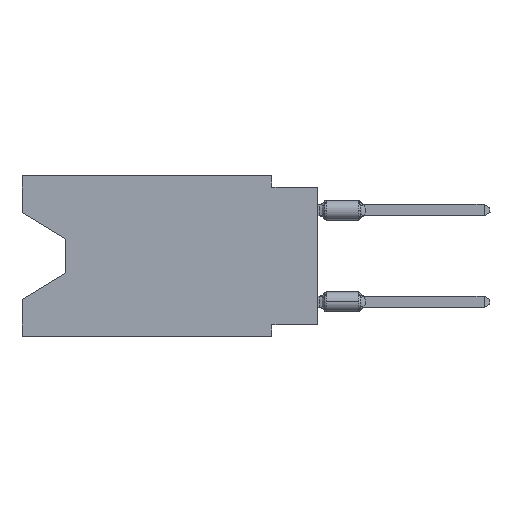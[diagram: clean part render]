
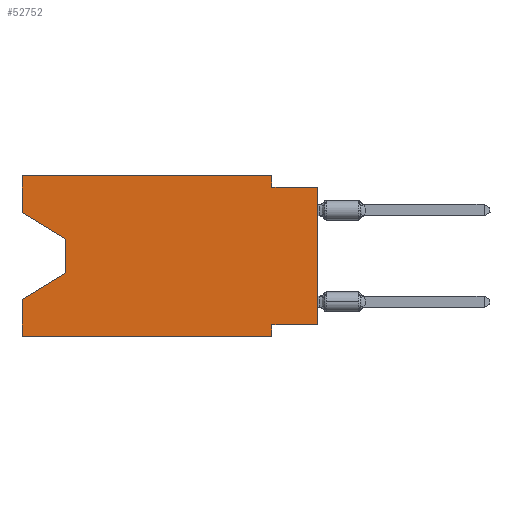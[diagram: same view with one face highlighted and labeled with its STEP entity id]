
A CAD part, left-side view. The second image highlights one B-rep face of the part: STEP entity #52752.
In plain terms, the highlighted planar face has unit normal (-1, 0, 0).
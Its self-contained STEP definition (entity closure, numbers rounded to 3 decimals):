
#1419 = VERTEX_POINT ( 'NONE', #22044 ) ;
#2936 = EDGE_CURVE ( 'NONE', #29716, #54374, #55581, .T. ) ;
#2951 = CARTESIAN_POINT ( 'NONE',  ( 0., 16.383, 0. ) ) ;
#3205 = VECTOR ( 'NONE', #17647, 1000. ) ;
#3366 = CARTESIAN_POINT ( 'NONE',  ( 0., 16.383, -8.89 ) ) ;
#3474 = LINE ( 'NONE', #35937, #59572 ) ;
#4101 = EDGE_CURVE ( 'NONE', #14996, #55507, #55052, .T. ) ;
#4157 = CARTESIAN_POINT ( 'NONE',  ( 0., 2.54, -8.89 ) ) ;
#6747 = ORIENTED_EDGE ( 'NONE', *, *, #42123, .F. ) ;
#6949 = ORIENTED_EDGE ( 'NONE', *, *, #49594, .F. ) ;
#8216 = EDGE_LOOP ( 'NONE', ( #9287, #29771, #29939, #52723, #46484, #22225, #6949, #10009, #47069, #6747, #33922, #58897 ) ) ;
#8384 = FACE_OUTER_BOUND ( 'NONE', #8216, .T. ) ;
#9071 = VECTOR ( 'NONE', #35763, 1000. ) ;
#9287 = ORIENTED_EDGE ( 'NONE', *, *, #38627, .T. ) ;
#10009 = ORIENTED_EDGE ( 'NONE', *, *, #59670, .T. ) ;
#11214 = EDGE_CURVE ( 'NONE', #1419, #29716, #36319, .T. ) ;
#11278 = CARTESIAN_POINT ( 'NONE',  ( 0., 16.383, -8.89 ) ) ;
#12383 = CARTESIAN_POINT ( 'NONE',  ( 0., 2.54, -8.255 ) ) ;
#12990 = LINE ( 'NONE', #50247, #9071 ) ;
#13232 = DIRECTION ( 'NONE',  ( 0., 0., -1. ) ) ;
#13260 = DIRECTION ( 'NONE',  ( 0., 0., 1. ) ) ;
#13549 = CARTESIAN_POINT ( 'NONE',  ( 0., 0., -0.635 ) ) ;
#14455 = EDGE_CURVE ( 'NONE', #52986, #44238, #45211, .T. ) ;
#14996 = VERTEX_POINT ( 'NONE', #30205 ) ;
#15705 = DIRECTION ( 'NONE',  ( 0., 0., -1. ) ) ;
#15811 = VERTEX_POINT ( 'NONE', #12383 ) ;
#16048 = VECTOR ( 'NONE', #13260, 1000. ) ;
#17647 = DIRECTION ( 'NONE',  ( 0., 0.855, -0.519 ) ) ;
#17855 = AXIS2_PLACEMENT_3D ( 'NONE', #44449, #21429, #13232 ) ;
#18126 = VERTEX_POINT ( 'NONE', #3366 ) ;
#18616 = VERTEX_POINT ( 'NONE', #4157 ) ;
#19093 = VECTOR ( 'NONE', #15705, 1000. ) ;
#19502 = CARTESIAN_POINT ( 'NONE',  ( 0., 16.383, -2.038 ) ) ;
#19797 = DIRECTION ( 'NONE',  ( 0., -0.855, -0.519 ) ) ;
#19832 = EDGE_CURVE ( 'NONE', #38888, #52986, #32906, .T. ) ;
#21429 = DIRECTION ( 'NONE',  ( 1., 0., 0. ) ) ;
#22044 = CARTESIAN_POINT ( 'NONE',  ( 0., 16.383, -2.038 ) ) ;
#22225 = ORIENTED_EDGE ( 'NONE', *, *, #54129, .F. ) ;
#22318 = PLANE ( 'NONE',  #17855 ) ;
#24357 = VECTOR ( 'NONE', #51919, 1000. ) ;
#25204 = DIRECTION ( 'NONE',  ( 0., -1., 0. ) ) ;
#26880 = VECTOR ( 'NONE', #25204, 1000. ) ;
#28217 = EDGE_CURVE ( 'NONE', #18126, #18616, #33749, .T. ) ;
#28597 = LINE ( 'NONE', #19502, #48849 ) ;
#28712 = VECTOR ( 'NONE', #47678, 1000. ) ;
#29716 = VERTEX_POINT ( 'NONE', #40355 ) ;
#29771 = ORIENTED_EDGE ( 'NONE', *, *, #19832, .T. ) ;
#29939 = ORIENTED_EDGE ( 'NONE', *, *, #14455, .T. ) ;
#30187 = CARTESIAN_POINT ( 'NONE',  ( 0., 13.97, -5.385 ) ) ;
#30205 = CARTESIAN_POINT ( 'NONE',  ( 0., 2.54, -0.635 ) ) ;
#32906 = LINE ( 'NONE', #33200, #28712 ) ;
#33200 = CARTESIAN_POINT ( 'NONE',  ( 0., 13.97, -3.505 ) ) ;
#33749 = LINE ( 'NONE', #11278, #26880 ) ;
#33922 = ORIENTED_EDGE ( 'NONE', *, *, #2936, .F. ) ;
#34188 = VECTOR ( 'NONE', #35529, 1000. ) ;
#35529 = DIRECTION ( 'NONE',  ( 0., 0., 1. ) ) ;
#35763 = DIRECTION ( 'NONE',  ( 0., 0., 1. ) ) ;
#35937 = CARTESIAN_POINT ( 'NONE',  ( 0., 2.54, -8.89 ) ) ;
#36319 = LINE ( 'NONE', #2951, #16048 ) ;
#37461 = CARTESIAN_POINT ( 'NONE',  ( 0., 0., -0.635 ) ) ;
#38627 = EDGE_CURVE ( 'NONE', #1419, #38888, #28597, .T. ) ;
#38888 = VERTEX_POINT ( 'NONE', #46308 ) ;
#39053 = LINE ( 'NONE', #39938, #53126 ) ;
#39938 = CARTESIAN_POINT ( 'NONE',  ( 0., 0., -8.255 ) ) ;
#40355 = CARTESIAN_POINT ( 'NONE',  ( 0., 16.383, 0. ) ) ;
#42039 = DIRECTION ( 'NONE',  ( 0., -1., 0. ) ) ;
#42123 = EDGE_CURVE ( 'NONE', #54374, #14996, #43880, .T. ) ;
#42581 = CARTESIAN_POINT ( 'NONE',  ( 0., 0., -8.255 ) ) ;
#43661 = EDGE_CURVE ( 'NONE', #18126, #44238, #12990, .T. ) ;
#43692 = CARTESIAN_POINT ( 'NONE',  ( 0., 0., 0. ) ) ;
#43880 = LINE ( 'NONE', #57215, #19093 ) ;
#44238 = VERTEX_POINT ( 'NONE', #51381 ) ;
#44449 = CARTESIAN_POINT ( 'NONE',  ( 0., 16.383, 0. ) ) ;
#45211 = LINE ( 'NONE', #30187, #3205 ) ;
#46308 = CARTESIAN_POINT ( 'NONE',  ( 0., 13.97, -3.505 ) ) ;
#46477 = CARTESIAN_POINT ( 'NONE',  ( 0., 16.383, 0. ) ) ;
#46484 = ORIENTED_EDGE ( 'NONE', *, *, #28217, .T. ) ;
#47069 = ORIENTED_EDGE ( 'NONE', *, *, #4101, .F. ) ;
#47678 = DIRECTION ( 'NONE',  ( 0., 0., -1. ) ) ;
#48849 = VECTOR ( 'NONE', #19797, 1000. ) ;
#49594 = EDGE_CURVE ( 'NONE', #56986, #15811, #39053, .T. ) ;
#50247 = CARTESIAN_POINT ( 'NONE',  ( 0., 16.383, 0. ) ) ;
#51381 = CARTESIAN_POINT ( 'NONE',  ( 0., 16.383, -6.852 ) ) ;
#51919 = DIRECTION ( 'NONE',  ( 0., -1., 0. ) ) ;
#52723 = ORIENTED_EDGE ( 'NONE', *, *, #43661, .F. ) ;
#52752 = ADVANCED_FACE ( 'NONE', ( #8384 ), #22318, .F. ) ;
#52780 = LINE ( 'NONE', #43692, #34188 ) ;
#52986 = VERTEX_POINT ( 'NONE', #59573 ) ;
#53126 = VECTOR ( 'NONE', #58403, 1000. ) ;
#53474 = VECTOR ( 'NONE', #42039, 1000. ) ;
#53796 = DIRECTION ( 'NONE',  ( 0., 0., -1. ) ) ;
#54129 = EDGE_CURVE ( 'NONE', #15811, #18616, #3474, .T. ) ;
#54374 = VERTEX_POINT ( 'NONE', #56419 ) ;
#55052 = LINE ( 'NONE', #13549, #53474 ) ;
#55507 = VERTEX_POINT ( 'NONE', #37461 ) ;
#55581 = LINE ( 'NONE', #46477, #24357 ) ;
#56419 = CARTESIAN_POINT ( 'NONE',  ( 0., 2.54, 0. ) ) ;
#56986 = VERTEX_POINT ( 'NONE', #42581 ) ;
#57215 = CARTESIAN_POINT ( 'NONE',  ( 0., 2.54, 0. ) ) ;
#58403 = DIRECTION ( 'NONE',  ( 0., 1., 0. ) ) ;
#58897 = ORIENTED_EDGE ( 'NONE', *, *, #11214, .F. ) ;
#59572 = VECTOR ( 'NONE', #53796, 1000. ) ;
#59573 = CARTESIAN_POINT ( 'NONE',  ( 0., 13.97, -5.385 ) ) ;
#59670 = EDGE_CURVE ( 'NONE', #56986, #55507, #52780, .T. ) ;
